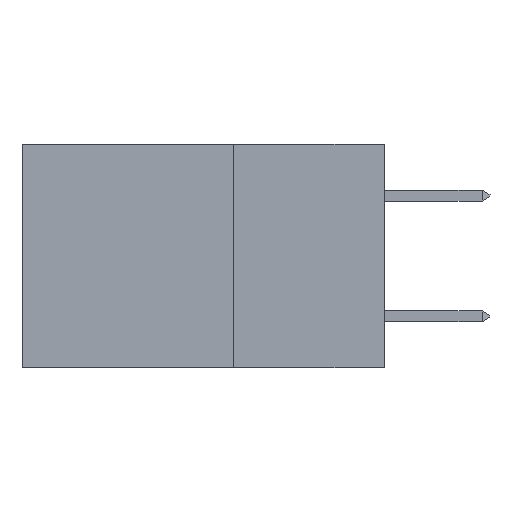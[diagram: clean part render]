
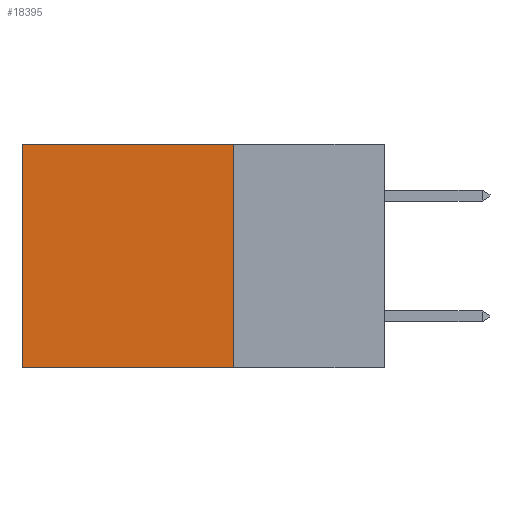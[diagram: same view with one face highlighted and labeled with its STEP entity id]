
A CAD part, left-side view. The second image highlights one B-rep face of the part: STEP entity #18395.
In plain terms, the highlighted planar face has unit normal (-1, 0, 0).
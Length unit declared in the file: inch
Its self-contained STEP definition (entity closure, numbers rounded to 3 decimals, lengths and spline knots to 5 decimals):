
#1072 = VECTOR ( 'NONE', #7222, 39.37008 ) ;
#1104 = CARTESIAN_POINT ( 'NONE',  ( 0.2875, 0.6, 0. ) ) ;
#3469 = AXIS2_PLACEMENT_3D ( 'NONE', #15109, #7364, #5914 ) ;
#5167 = EDGE_CURVE ( 'NONE', #18655, #8279, #11175, .T. ) ;
#5914 = DIRECTION ( 'NONE',  ( 0., 0., -1. ) ) ;
#6607 = LINE ( 'NONE', #9279, #18526 ) ;
#6673 = LINE ( 'NONE', #16096, #1072 ) ;
#7125 = VECTOR ( 'NONE', #17951, 39.37008 ) ;
#7222 = DIRECTION ( 'NONE',  ( 0., 1., 0. ) ) ;
#7364 = DIRECTION ( 'NONE',  ( 1., 0., 0. ) ) ;
#7760 = DIRECTION ( 'NONE',  ( 0., 0., -1. ) ) ;
#8279 = VERTEX_POINT ( 'NONE', #18384 ) ;
#8879 = VERTEX_POINT ( 'NONE', #9170 ) ;
#9170 = CARTESIAN_POINT ( 'NONE',  ( 0.2875, 0.6, 0. ) ) ;
#9233 = ORIENTED_EDGE ( 'NONE', *, *, #5167, .F. ) ;
#9279 = CARTESIAN_POINT ( 'NONE',  ( 0.2875, 0.25, 0. ) ) ;
#10075 = EDGE_CURVE ( 'NONE', #15159, #8879, #6673, .T. ) ;
#10509 = EDGE_CURVE ( 'NONE', #8879, #8279, #10636, .T. ) ;
#10636 = LINE ( 'NONE', #1104, #7125 ) ;
#10993 = EDGE_LOOP ( 'NONE', ( #12140, #9233, #17922, #19017 ) ) ;
#11175 = LINE ( 'NONE', #16930, #16073 ) ;
#12140 = ORIENTED_EDGE ( 'NONE', *, *, #10509, .T. ) ;
#13621 = PLANE ( 'NONE',  #3469 ) ;
#14217 = DIRECTION ( 'NONE',  ( 0., 1., 0. ) ) ;
#15109 = CARTESIAN_POINT ( 'NONE',  ( 0.2875, 0.25, 0. ) ) ;
#15159 = VERTEX_POINT ( 'NONE', #17015 ) ;
#16073 = VECTOR ( 'NONE', #14217, 39.37008 ) ;
#16096 = CARTESIAN_POINT ( 'NONE',  ( 0.2875, 0.25, 0. ) ) ;
#16927 = CARTESIAN_POINT ( 'NONE',  ( 0.2875, 0.25, -0.37 ) ) ;
#16930 = CARTESIAN_POINT ( 'NONE',  ( 0.2875, 0.25, -0.37 ) ) ;
#17015 = CARTESIAN_POINT ( 'NONE',  ( 0.2875, 0.25, 0. ) ) ;
#17761 = EDGE_CURVE ( 'NONE', #15159, #18655, #6607, .T. ) ;
#17922 = ORIENTED_EDGE ( 'NONE', *, *, #17761, .F. ) ;
#17951 = DIRECTION ( 'NONE',  ( 0., 0., -1. ) ) ;
#18266 = FACE_OUTER_BOUND ( 'NONE', #10993, .T. ) ;
#18384 = CARTESIAN_POINT ( 'NONE',  ( 0.2875, 0.6, -0.37 ) ) ;
#18395 = ADVANCED_FACE ( 'NONE', ( #18266 ), #13621, .F. ) ;
#18526 = VECTOR ( 'NONE', #7760, 39.37008 ) ;
#18655 = VERTEX_POINT ( 'NONE', #16927 ) ;
#19017 = ORIENTED_EDGE ( 'NONE', *, *, #10075, .T. ) ;
